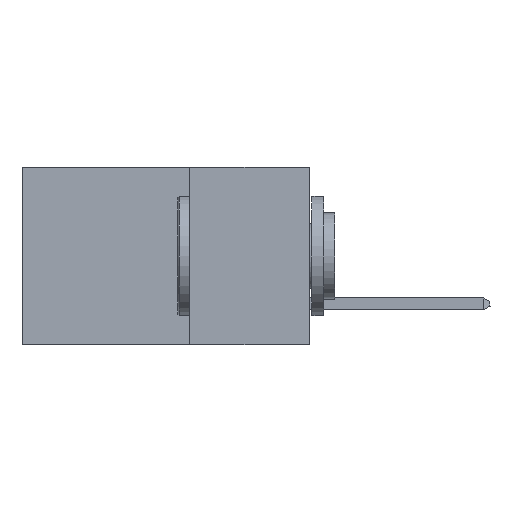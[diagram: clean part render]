
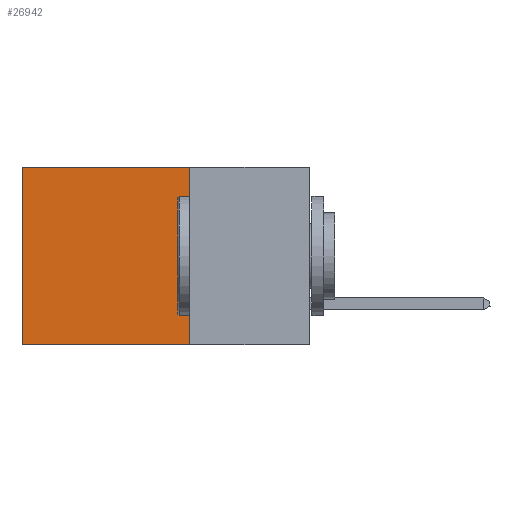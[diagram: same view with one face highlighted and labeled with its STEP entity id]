
A CAD part, left-side view. The second image highlights one B-rep face of the part: STEP entity #26942.
In plain terms, the highlighted planar face has unit normal (-1, 0, 0).
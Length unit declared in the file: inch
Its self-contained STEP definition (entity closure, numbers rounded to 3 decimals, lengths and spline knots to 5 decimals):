
#1353 = LINE ( 'NONE', #16422, #28176 ) ;
#1519 = VECTOR ( 'NONE', #22000, 39.37008 ) ;
#1667 = DIRECTION ( 'NONE',  ( 1., 0., 0. ) ) ;
#1761 = CARTESIAN_POINT ( 'NONE',  ( 0.2875, 0.25, 0. ) ) ;
#2210 = VERTEX_POINT ( 'NONE', #1761 ) ;
#2238 = DIRECTION ( 'NONE',  ( 0., 1., 0. ) ) ;
#2517 = VERTEX_POINT ( 'NONE', #18291 ) ;
#4063 = LINE ( 'NONE', #20367, #1519 ) ;
#4131 = CARTESIAN_POINT ( 'NONE',  ( 0.2875, 0.25, -0.37 ) ) ;
#5511 = CARTESIAN_POINT ( 'NONE',  ( 0.2875, 0.6, 0. ) ) ;
#6226 = EDGE_CURVE ( 'NONE', #32943, #2517, #4063, .T. ) ;
#6436 = EDGE_CURVE ( 'NONE', #2210, #32943, #23747, .T. ) ;
#7324 = FACE_OUTER_BOUND ( 'NONE', #30686, .T. ) ;
#7673 = AXIS2_PLACEMENT_3D ( 'NONE', #23105, #1667, #31368 ) ;
#8116 = ORIENTED_EDGE ( 'NONE', *, *, #16330, .T. ) ;
#10828 = VECTOR ( 'NONE', #14154, 39.37008 ) ;
#11441 = CARTESIAN_POINT ( 'NONE',  ( 0.2875, 0.25, 0. ) ) ;
#14154 = DIRECTION ( 'NONE',  ( 0., 0., -1. ) ) ;
#16330 = EDGE_CURVE ( 'NONE', #26491, #2517, #1353, .T. ) ;
#16422 = CARTESIAN_POINT ( 'NONE',  ( 0.2875, 0.6, 0. ) ) ;
#16768 = DIRECTION ( 'NONE',  ( 0., 0., -1. ) ) ;
#17910 = LINE ( 'NONE', #23560, #31322 ) ;
#18150 = ORIENTED_EDGE ( 'NONE', *, *, #6436, .F. ) ;
#18291 = CARTESIAN_POINT ( 'NONE',  ( 0.2875, 0.6, -0.37 ) ) ;
#20367 = CARTESIAN_POINT ( 'NONE',  ( 0.2875, 0.25, -0.37 ) ) ;
#20800 = PLANE ( 'NONE',  #7673 ) ;
#22000 = DIRECTION ( 'NONE',  ( 0., 1., 0. ) ) ;
#23105 = CARTESIAN_POINT ( 'NONE',  ( 0.2875, 0.25, 0. ) ) ;
#23560 = CARTESIAN_POINT ( 'NONE',  ( 0.2875, 0.25, 0. ) ) ;
#23747 = LINE ( 'NONE', #11441, #10828 ) ;
#26491 = VERTEX_POINT ( 'NONE', #5511 ) ;
#26942 = ADVANCED_FACE ( 'NONE', ( #7324 ), #20800, .F. ) ;
#27241 = ORIENTED_EDGE ( 'NONE', *, *, #28264, .T. ) ;
#28176 = VECTOR ( 'NONE', #16768, 39.37008 ) ;
#28264 = EDGE_CURVE ( 'NONE', #2210, #26491, #17910, .T. ) ;
#30686 = EDGE_LOOP ( 'NONE', ( #8116, #33771, #18150, #27241 ) ) ;
#31322 = VECTOR ( 'NONE', #2238, 39.37008 ) ;
#31368 = DIRECTION ( 'NONE',  ( 0., 0., -1. ) ) ;
#32943 = VERTEX_POINT ( 'NONE', #4131 ) ;
#33771 = ORIENTED_EDGE ( 'NONE', *, *, #6226, .F. ) ;
